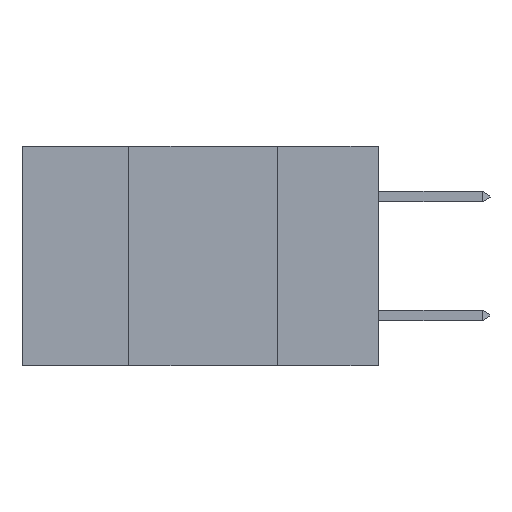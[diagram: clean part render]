
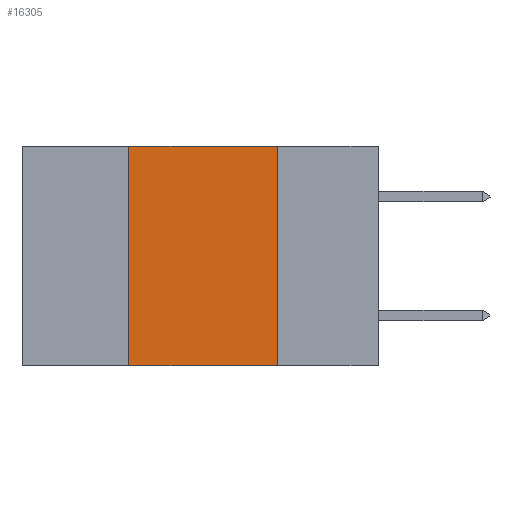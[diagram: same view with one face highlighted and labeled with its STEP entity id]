
A CAD part, left-side view. The second image highlights one B-rep face of the part: STEP entity #16305.
In plain terms, the highlighted planar face has unit normal (-1, 0, 0).
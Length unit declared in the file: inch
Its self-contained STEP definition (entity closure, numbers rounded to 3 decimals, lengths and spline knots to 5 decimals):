
#481 = LINE ( 'NONE', #19754, #9434 ) ;
#973 = CARTESIAN_POINT ( 'NONE',  ( 0., 0.6, 0. ) ) ;
#993 = CARTESIAN_POINT ( 'NONE',  ( 0., 0.17, 0. ) ) ;
#1892 = VERTEX_POINT ( 'NONE', #993 ) ;
#2707 = CARTESIAN_POINT ( 'NONE',  ( 0., 0.42, 0. ) ) ;
#2723 = DIRECTION ( 'NONE',  ( 0., 0., -1. ) ) ;
#3105 = CARTESIAN_POINT ( 'NONE',  ( 0., 0.17, -0.37 ) ) ;
#3181 = EDGE_CURVE ( 'NONE', #1892, #15576, #481, .T. ) ;
#5300 = AXIS2_PLACEMENT_3D ( 'NONE', #973, #12551, #2723 ) ;
#5838 = VECTOR ( 'NONE', #11013, 39.37008 ) ;
#6130 = CARTESIAN_POINT ( 'NONE',  ( 0., 0.42, 0. ) ) ;
#6513 = DIRECTION ( 'NONE',  ( 0., -1., 0. ) ) ;
#6551 = LINE ( 'NONE', #19147, #16083 ) ;
#6560 = EDGE_LOOP ( 'NONE', ( #18773, #15561, #11592, #20017 ) ) ;
#7705 = PLANE ( 'NONE',  #5300 ) ;
#8421 = LINE ( 'NONE', #19308, #12667 ) ;
#8699 = VERTEX_POINT ( 'NONE', #20523 ) ;
#9434 = VECTOR ( 'NONE', #19772, 39.37008 ) ;
#9660 = DIRECTION ( 'NONE',  ( 0., -1., 0. ) ) ;
#10218 = LINE ( 'NONE', #2707, #5838 ) ;
#10349 = EDGE_CURVE ( 'NONE', #8699, #15576, #8421, .T. ) ;
#11013 = DIRECTION ( 'NONE',  ( 0., 0., 1. ) ) ;
#11592 = ORIENTED_EDGE ( 'NONE', *, *, #20852, .F. ) ;
#12551 = DIRECTION ( 'NONE',  ( 1., 0., 0. ) ) ;
#12667 = VECTOR ( 'NONE', #6513, 39.37008 ) ;
#13542 = VERTEX_POINT ( 'NONE', #6130 ) ;
#15512 = EDGE_CURVE ( 'NONE', #13542, #1892, #6551, .T. ) ;
#15561 = ORIENTED_EDGE ( 'NONE', *, *, #15512, .F. ) ;
#15576 = VERTEX_POINT ( 'NONE', #3105 ) ;
#16083 = VECTOR ( 'NONE', #9660, 39.37008 ) ;
#16305 = ADVANCED_FACE ( 'NONE', ( #20259 ), #7705, .F. ) ;
#18773 = ORIENTED_EDGE ( 'NONE', *, *, #3181, .F. ) ;
#19147 = CARTESIAN_POINT ( 'NONE',  ( 0., 0.6, 0. ) ) ;
#19308 = CARTESIAN_POINT ( 'NONE',  ( 0., 0.6, -0.37 ) ) ;
#19754 = CARTESIAN_POINT ( 'NONE',  ( 0., 0.17, 0. ) ) ;
#19772 = DIRECTION ( 'NONE',  ( 0., 0., -1. ) ) ;
#20017 = ORIENTED_EDGE ( 'NONE', *, *, #10349, .T. ) ;
#20259 = FACE_OUTER_BOUND ( 'NONE', #6560, .T. ) ;
#20523 = CARTESIAN_POINT ( 'NONE',  ( 0., 0.42, -0.37 ) ) ;
#20852 = EDGE_CURVE ( 'NONE', #8699, #13542, #10218, .T. ) ;
